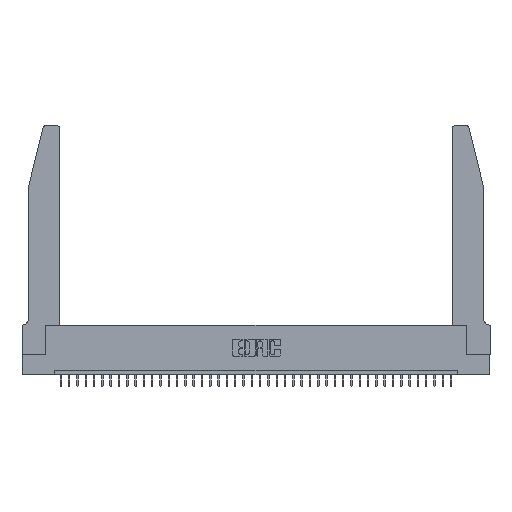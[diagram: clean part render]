
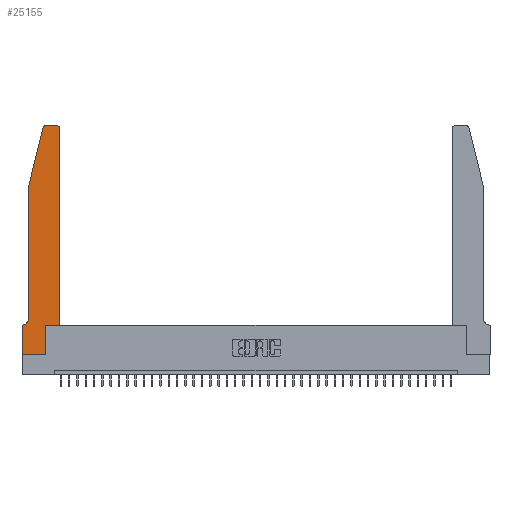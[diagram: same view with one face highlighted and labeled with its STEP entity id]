
A CAD part, top view. The second image highlights one B-rep face of the part: STEP entity #25155.
In plain terms, the highlighted planar face has unit normal (0, 0, 1).
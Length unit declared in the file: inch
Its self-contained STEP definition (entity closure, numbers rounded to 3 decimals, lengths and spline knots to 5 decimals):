
#142 = AXIS2_PLACEMENT_3D ( 'NONE', #26658, #21140, #1492 ) ;
#176 = CARTESIAN_POINT ( 'NONE',  ( 0.4205, 2.72, 0.37 ) ) ;
#720 = DIRECTION ( 'NONE',  ( 1., 0., 0. ) ) ;
#1050 = LINE ( 'NONE', #31765, #11036 ) ;
#1492 = DIRECTION ( 'NONE',  ( 1., 0., 0. ) ) ;
#1545 = ORIENTED_EDGE ( 'NONE', *, *, #2086, .T. ) ;
#1892 = VECTOR ( 'NONE', #30379, 39.37008 ) ;
#2086 = EDGE_CURVE ( 'NONE', #11879, #16389, #25699, .T. ) ;
#2104 = ORIENTED_EDGE ( 'NONE', *, *, #25414, .T. ) ;
#2106 = CARTESIAN_POINT ( 'NONE',  ( 0.0055, 0.42, 0.37 ) ) ;
#2712 = DIRECTION ( 'NONE',  ( -1., 0., 0. ) ) ;
#3671 = DIRECTION ( 'NONE',  ( -1., 0., 0. ) ) ;
#3723 = VERTEX_POINT ( 'NONE', #10256 ) ;
#4139 = CIRCLE ( 'NONE', #10673, 0.03 ) ;
#4262 = CARTESIAN_POINT ( 'NONE',  ( 0.25487, 2.72718, 0.37 ) ) ;
#5748 = ORIENTED_EDGE ( 'NONE', *, *, #33197, .T. ) ;
#6035 = DIRECTION ( 'NONE',  ( 0., 1., 0. ) ) ;
#6658 = EDGE_LOOP ( 'NONE', ( #38151, #26336, #5748, #25235, #2104, #26258, #28929, #1545, #29602, #16730, #10326, #10296 ) ) ;
#6871 = CARTESIAN_POINT ( 'NONE',  ( 0., 0., 0.37 ) ) ;
#6908 = LINE ( 'NONE', #19703, #10940 ) ;
#7155 = VERTEX_POINT ( 'NONE', #4262 ) ;
#7290 = CARTESIAN_POINT ( 'NONE',  ( 0.0055, 0.35, 0.37 ) ) ;
#7739 = VECTOR ( 'NONE', #6035, 39.37008 ) ;
#7781 = VERTEX_POINT ( 'NONE', #9832 ) ;
#8324 = CIRCLE ( 'NONE', #35584, 0.07 ) ;
#9305 = FACE_OUTER_BOUND ( 'NONE', #6658, .T. ) ;
#9323 = EDGE_CURVE ( 'NONE', #7781, #15233, #33027, .T. ) ;
#9501 = CARTESIAN_POINT ( 'NONE',  ( 0., 0.35, 0.37 ) ) ;
#9720 = EDGE_CURVE ( 'NONE', #34010, #3723, #1050, .T. ) ;
#9780 = LINE ( 'NONE', #13413, #19116 ) ;
#9796 = LINE ( 'NONE', #19528, #22207 ) ;
#9832 = CARTESIAN_POINT ( 'NONE',  ( 0.0755, 2., 0.37 ) ) ;
#9949 = VECTOR ( 'NONE', #24523, 39.37008 ) ;
#10095 = DIRECTION ( 'NONE',  ( 1., 0., 0. ) ) ;
#10163 = VERTEX_POINT ( 'NONE', #38408 ) ;
#10256 = CARTESIAN_POINT ( 'NONE',  ( 0.284, 2.75, 0.37 ) ) ;
#10296 = ORIENTED_EDGE ( 'NONE', *, *, #32550, .T. ) ;
#10326 = ORIENTED_EDGE ( 'NONE', *, *, #29862, .T. ) ;
#10673 = AXIS2_PLACEMENT_3D ( 'NONE', #176, #28194, #27986 ) ;
#10940 = VECTOR ( 'NONE', #31720, 39.37008 ) ;
#11036 = VECTOR ( 'NONE', #28459, 39.37008 ) ;
#11840 = CIRCLE ( 'NONE', #142, 0.03 ) ;
#11879 = VERTEX_POINT ( 'NONE', #6871 ) ;
#11929 = LINE ( 'NONE', #21663, #7739 ) ;
#12462 = CARTESIAN_POINT ( 'NONE',  ( 0.0755, 0.42, 0.37 ) ) ;
#13129 = VERTEX_POINT ( 'NONE', #18029 ) ;
#13192 = EDGE_CURVE ( 'NONE', #16389, #38042, #11929, .T. ) ;
#13206 = DIRECTION ( 'NONE',  ( -0.239, -0.971, 0. ) ) ;
#13413 = CARTESIAN_POINT ( 'NONE',  ( 0.0755, 2., 0.37 ) ) ;
#14477 = VERTEX_POINT ( 'NONE', #7290 ) ;
#15233 = VERTEX_POINT ( 'NONE', #12462 ) ;
#16389 = VERTEX_POINT ( 'NONE', #25853 ) ;
#16730 = ORIENTED_EDGE ( 'NONE', *, *, #19026, .T. ) ;
#18029 = CARTESIAN_POINT ( 'NONE',  ( 0., 0.35, 0.37 ) ) ;
#18404 = CARTESIAN_POINT ( 'NONE',  ( 0.4505, 2.72, 0.37 ) ) ;
#19026 = EDGE_CURVE ( 'NONE', #38042, #10163, #31063, .T. ) ;
#19116 = VECTOR ( 'NONE', #13206, 39.37008 ) ;
#19334 = VERTEX_POINT ( 'NONE', #18404 ) ;
#19528 = CARTESIAN_POINT ( 'NONE',  ( 0.0755, 0.35, 0.37 ) ) ;
#19703 = CARTESIAN_POINT ( 'NONE',  ( 0., 0., 0.37 ) ) ;
#21011 = CARTESIAN_POINT ( 'NONE',  ( 0.0755, 2., 0.37 ) ) ;
#21140 = DIRECTION ( 'NONE',  ( 0., 0., 1. ) ) ;
#21663 = CARTESIAN_POINT ( 'NONE',  ( 0.2865, 0.35, 0.37 ) ) ;
#22207 = VECTOR ( 'NONE', #3671, 39.37008 ) ;
#24523 = DIRECTION ( 'NONE',  ( 1., 0., 0. ) ) ;
#25155 = ADVANCED_FACE ( 'NONE', ( #9305 ), #37531, .T. ) ;
#25235 = ORIENTED_EDGE ( 'NONE', *, *, #9323, .T. ) ;
#25414 = EDGE_CURVE ( 'NONE', #15233, #14477, #8324, .T. ) ;
#25699 = LINE ( 'NONE', #31843, #39786 ) ;
#25853 = CARTESIAN_POINT ( 'NONE',  ( 0.2865, 0., 0.37 ) ) ;
#26258 = ORIENTED_EDGE ( 'NONE', *, *, #28982, .T. ) ;
#26336 = ORIENTED_EDGE ( 'NONE', *, *, #28917, .T. ) ;
#26658 = CARTESIAN_POINT ( 'NONE',  ( 0.284, 2.72, 0.37 ) ) ;
#27986 = DIRECTION ( 'NONE',  ( 1., 0., 0. ) ) ;
#28194 = DIRECTION ( 'NONE',  ( 0., 0., 1. ) ) ;
#28459 = DIRECTION ( 'NONE',  ( -1., 0., 0. ) ) ;
#28917 = EDGE_CURVE ( 'NONE', #3723, #7155, #11840, .T. ) ;
#28929 = ORIENTED_EDGE ( 'NONE', *, *, #39595, .T. ) ;
#28982 = EDGE_CURVE ( 'NONE', #14477, #13129, #9796, .T. ) ;
#29069 = AXIS2_PLACEMENT_3D ( 'NONE', #9501, #37936, #10095 ) ;
#29602 = ORIENTED_EDGE ( 'NONE', *, *, #13192, .T. ) ;
#29862 = EDGE_CURVE ( 'NONE', #10163, #19334, #38946, .T. ) ;
#30067 = VECTOR ( 'NONE', #36329, 39.37008 ) ;
#30379 = DIRECTION ( 'NONE',  ( 0., -1., 0. ) ) ;
#30594 = DIRECTION ( 'NONE',  ( 0., 0., -1. ) ) ;
#31063 = LINE ( 'NONE', #39579, #9949 ) ;
#31720 = DIRECTION ( 'NONE',  ( 0., -1., 0. ) ) ;
#31765 = CARTESIAN_POINT ( 'NONE',  ( 0.2605, 2.75, 0.37 ) ) ;
#31843 = CARTESIAN_POINT ( 'NONE',  ( 0., 0., 0.37 ) ) ;
#32550 = EDGE_CURVE ( 'NONE', #19334, #34010, #4139, .T. ) ;
#33027 = LINE ( 'NONE', #21011, #1892 ) ;
#33197 = EDGE_CURVE ( 'NONE', #7155, #7781, #9780, .T. ) ;
#34010 = VERTEX_POINT ( 'NONE', #39542 ) ;
#35584 = AXIS2_PLACEMENT_3D ( 'NONE', #2106, #30594, #2712 ) ;
#36329 = DIRECTION ( 'NONE',  ( 0., 1., 0. ) ) ;
#37531 = PLANE ( 'NONE',  #29069 ) ;
#37651 = CARTESIAN_POINT ( 'NONE',  ( 0.2865, 0.35, 0.37 ) ) ;
#37936 = DIRECTION ( 'NONE',  ( 0., 0., 1. ) ) ;
#38042 = VERTEX_POINT ( 'NONE', #37651 ) ;
#38151 = ORIENTED_EDGE ( 'NONE', *, *, #9720, .T. ) ;
#38408 = CARTESIAN_POINT ( 'NONE',  ( 0.4505, 0.35, 0.37 ) ) ;
#38565 = CARTESIAN_POINT ( 'NONE',  ( 0.4505, 0.35, 0.37 ) ) ;
#38946 = LINE ( 'NONE', #38565, #30067 ) ;
#39542 = CARTESIAN_POINT ( 'NONE',  ( 0.4205, 2.75, 0.37 ) ) ;
#39579 = CARTESIAN_POINT ( 'NONE',  ( 0.4505, 0.35, 0.37 ) ) ;
#39595 = EDGE_CURVE ( 'NONE', #13129, #11879, #6908, .T. ) ;
#39786 = VECTOR ( 'NONE', #720, 39.37008 ) ;
